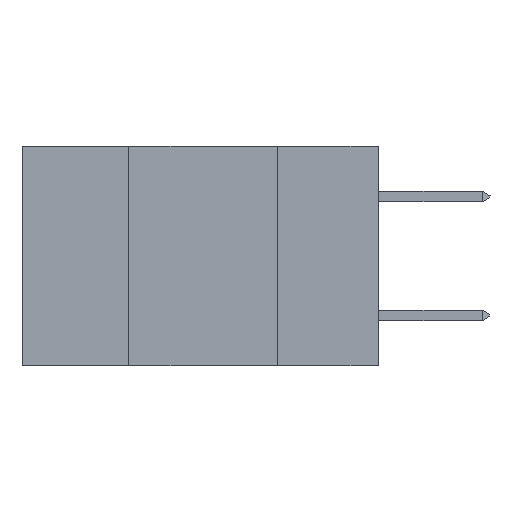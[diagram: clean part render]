
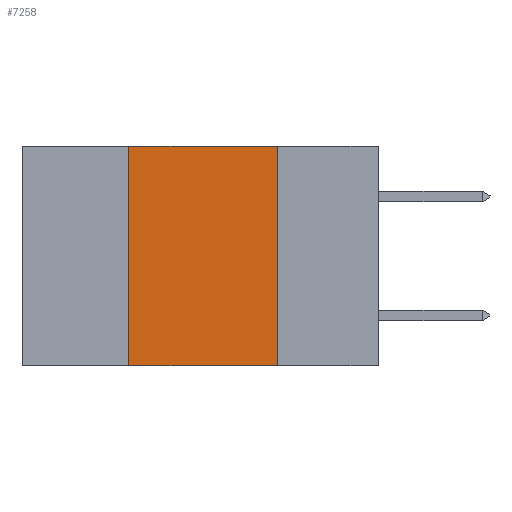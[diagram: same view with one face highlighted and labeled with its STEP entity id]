
A CAD part, left-side view. The second image highlights one B-rep face of the part: STEP entity #7258.
In plain terms, the highlighted planar face has unit normal (-1, 0, 0).
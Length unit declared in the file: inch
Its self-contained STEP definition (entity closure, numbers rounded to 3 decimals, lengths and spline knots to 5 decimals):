
#669 = DIRECTION ( 'NONE',  ( 0., 0., -1. ) ) ;
#1012 = FACE_OUTER_BOUND ( 'NONE', #10935, .T. ) ;
#1014 = VERTEX_POINT ( 'NONE', #11163 ) ;
#1459 = VERTEX_POINT ( 'NONE', #4107 ) ;
#3132 = LINE ( 'NONE', #9897, #8066 ) ;
#3371 = EDGE_CURVE ( 'NONE', #7366, #1459, #7011, .T. ) ;
#3433 = ORIENTED_EDGE ( 'NONE', *, *, #3371, .F. ) ;
#3693 = DIRECTION ( 'NONE',  ( 0., 0., -1. ) ) ;
#3726 = DIRECTION ( 'NONE',  ( 0., 0., 1. ) ) ;
#3794 = VECTOR ( 'NONE', #10736, 39.37008 ) ;
#4107 = CARTESIAN_POINT ( 'NONE',  ( 0., 0.17, 0. ) ) ;
#4515 = DIRECTION ( 'NONE',  ( 1., 0., 0. ) ) ;
#4653 = DIRECTION ( 'NONE',  ( 0., -1., 0. ) ) ;
#4677 = CARTESIAN_POINT ( 'NONE',  ( 0., 0.42, -0.37 ) ) ;
#6004 = ORIENTED_EDGE ( 'NONE', *, *, #8618, .T. ) ;
#7011 = LINE ( 'NONE', #7073, #3794 ) ;
#7030 = PLANE ( 'NONE',  #10180 ) ;
#7070 = LINE ( 'NONE', #4677, #10411 ) ;
#7073 = CARTESIAN_POINT ( 'NONE',  ( 0., 0.6, 0. ) ) ;
#7258 = ADVANCED_FACE ( 'NONE', ( #1012 ), #7030, .F. ) ;
#7366 = VERTEX_POINT ( 'NONE', #7545 ) ;
#7545 = CARTESIAN_POINT ( 'NONE',  ( 0., 0.42, 0. ) ) ;
#7550 = CARTESIAN_POINT ( 'NONE',  ( 0., 0.17, -0.37 ) ) ;
#7695 = ORIENTED_EDGE ( 'NONE', *, *, #9408, .F. ) ;
#8049 = CARTESIAN_POINT ( 'NONE',  ( 0., 0.6, 0. ) ) ;
#8066 = VECTOR ( 'NONE', #4653, 39.37008 ) ;
#8618 = EDGE_CURVE ( 'NONE', #1014, #9993, #3132, .T. ) ;
#9408 = EDGE_CURVE ( 'NONE', #1014, #7366, #7070, .T. ) ;
#9897 = CARTESIAN_POINT ( 'NONE',  ( 0., 0.6, -0.37 ) ) ;
#9993 = VERTEX_POINT ( 'NONE', #10012 ) ;
#10012 = CARTESIAN_POINT ( 'NONE',  ( 0., 0.17, -0.37 ) ) ;
#10089 = ORIENTED_EDGE ( 'NONE', *, *, #10627, .F. ) ;
#10180 = AXIS2_PLACEMENT_3D ( 'NONE', #8049, #4515, #3693 ) ;
#10326 = VECTOR ( 'NONE', #669, 39.37008 ) ;
#10411 = VECTOR ( 'NONE', #3726, 39.37008 ) ;
#10627 = EDGE_CURVE ( 'NONE', #1459, #9993, #11104, .T. ) ;
#10736 = DIRECTION ( 'NONE',  ( 0., -1., 0. ) ) ;
#10935 = EDGE_LOOP ( 'NONE', ( #10089, #3433, #7695, #6004 ) ) ;
#11104 = LINE ( 'NONE', #7550, #10326 ) ;
#11163 = CARTESIAN_POINT ( 'NONE',  ( 0., 0.42, -0.37 ) ) ;
